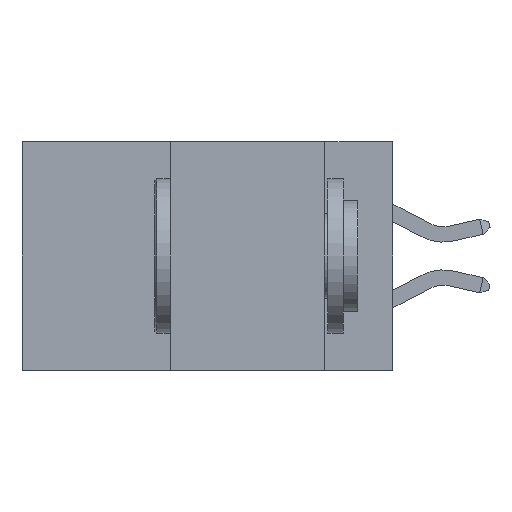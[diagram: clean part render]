
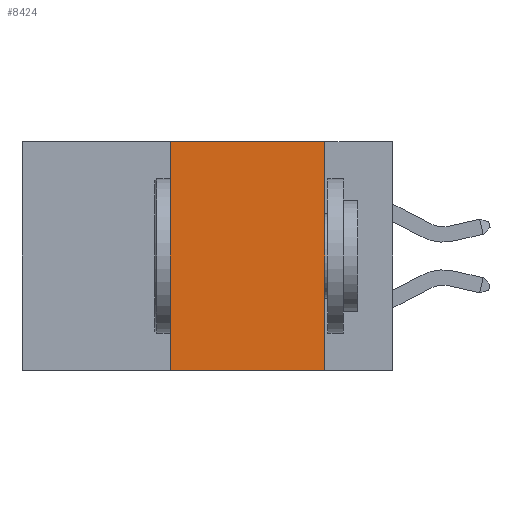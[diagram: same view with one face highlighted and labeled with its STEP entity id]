
A CAD part, left-side view. The second image highlights one B-rep face of the part: STEP entity #8424.
In plain terms, the highlighted planar face has unit normal (-1, 0, 0).
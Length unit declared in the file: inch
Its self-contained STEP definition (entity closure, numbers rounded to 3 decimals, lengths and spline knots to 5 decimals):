
#294 = CARTESIAN_POINT ( 'NONE',  ( 0., 0.11, 0. ) ) ;
#871 = ORIENTED_EDGE ( 'NONE', *, *, #7014, .F. ) ;
#1309 = ORIENTED_EDGE ( 'NONE', *, *, #9986, .F. ) ;
#1421 = ORIENTED_EDGE ( 'NONE', *, *, #6454, .F. ) ;
#1739 = LINE ( 'NONE', #8539, #6114 ) ;
#2054 = CARTESIAN_POINT ( 'NONE',  ( 0., 0.11, 0. ) ) ;
#2847 = DIRECTION ( 'NONE',  ( 0., -1., 0. ) ) ;
#2855 = VECTOR ( 'NONE', #2847, 39.37008 ) ;
#2861 = VERTEX_POINT ( 'NONE', #9843 ) ;
#4076 = PLANE ( 'NONE',  #10699 ) ;
#4946 = FACE_OUTER_BOUND ( 'NONE', #6285, .T. ) ;
#5277 = CARTESIAN_POINT ( 'NONE',  ( 0., 0.36, 0. ) ) ;
#5440 = LINE ( 'NONE', #294, #7678 ) ;
#5914 = DIRECTION ( 'NONE',  ( 0., 0., -1. ) ) ;
#6114 = VECTOR ( 'NONE', #9438, 39.37008 ) ;
#6185 = VERTEX_POINT ( 'NONE', #7706 ) ;
#6264 = DIRECTION ( 'NONE',  ( 0., 0., 1. ) ) ;
#6285 = EDGE_LOOP ( 'NONE', ( #871, #1309, #1421, #8490 ) ) ;
#6454 = EDGE_CURVE ( 'NONE', #11567, #2861, #8860, .T. ) ;
#6761 = CARTESIAN_POINT ( 'NONE',  ( 0., 0.36, -0.37 ) ) ;
#7014 = EDGE_CURVE ( 'NONE', #10012, #6185, #5440, .T. ) ;
#7678 = VECTOR ( 'NONE', #8796, 39.37008 ) ;
#7690 = VECTOR ( 'NONE', #6264, 39.37008 ) ;
#7706 = CARTESIAN_POINT ( 'NONE',  ( 0., 0.11, -0.37 ) ) ;
#7793 = CARTESIAN_POINT ( 'NONE',  ( 0., 0.6, 0. ) ) ;
#8424 = ADVANCED_FACE ( 'NONE', ( #4946 ), #4076, .F. ) ;
#8490 = ORIENTED_EDGE ( 'NONE', *, *, #8792, .T. ) ;
#8539 = CARTESIAN_POINT ( 'NONE',  ( 0., 0.6, 0. ) ) ;
#8792 = EDGE_CURVE ( 'NONE', #11567, #6185, #9922, .T. ) ;
#8796 = DIRECTION ( 'NONE',  ( 0., 0., -1. ) ) ;
#8860 = LINE ( 'NONE', #5277, #7690 ) ;
#9314 = CARTESIAN_POINT ( 'NONE',  ( 0., 0.6, -0.37 ) ) ;
#9438 = DIRECTION ( 'NONE',  ( 0., -1., 0. ) ) ;
#9843 = CARTESIAN_POINT ( 'NONE',  ( 0., 0.36, 0. ) ) ;
#9922 = LINE ( 'NONE', #9314, #2855 ) ;
#9986 = EDGE_CURVE ( 'NONE', #2861, #10012, #1739, .T. ) ;
#10012 = VERTEX_POINT ( 'NONE', #2054 ) ;
#10699 = AXIS2_PLACEMENT_3D ( 'NONE', #7793, #11298, #5914 ) ;
#11298 = DIRECTION ( 'NONE',  ( 1., 0., 0. ) ) ;
#11567 = VERTEX_POINT ( 'NONE', #6761 ) ;
